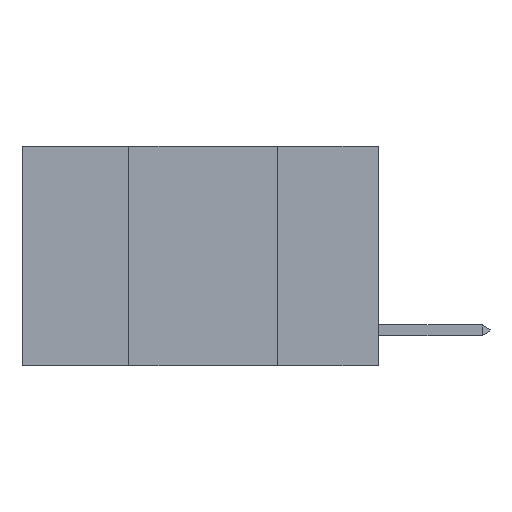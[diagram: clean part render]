
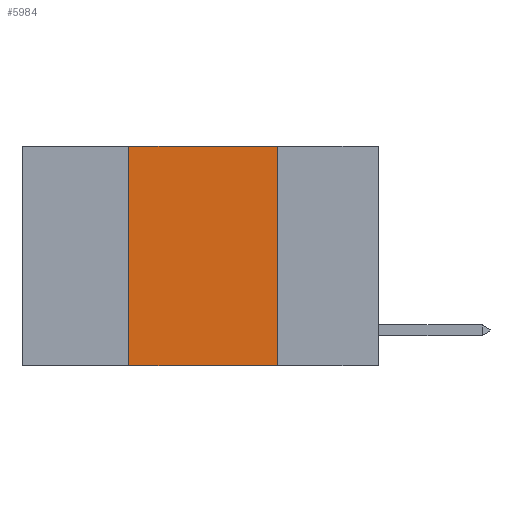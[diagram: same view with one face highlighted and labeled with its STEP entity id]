
A CAD part, left-side view. The second image highlights one B-rep face of the part: STEP entity #5984.
In plain terms, the highlighted planar face has unit normal (-1, 0, 0).
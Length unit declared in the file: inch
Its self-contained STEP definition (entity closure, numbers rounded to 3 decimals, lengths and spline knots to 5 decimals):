
#503 = DIRECTION ( 'NONE',  ( 0., 0., 1. ) ) ;
#614 = VECTOR ( 'NONE', #2839, 39.37008 ) ;
#666 = DIRECTION ( 'NONE',  ( 0., -1., 0. ) ) ;
#757 = CARTESIAN_POINT ( 'NONE',  ( 0., 0.6, 0. ) ) ;
#1487 = EDGE_CURVE ( 'NONE', #12241, #12350, #9036, .T. ) ;
#1735 = CARTESIAN_POINT ( 'NONE',  ( 0., 0.42, -0.37 ) ) ;
#2281 = LINE ( 'NONE', #3806, #614 ) ;
#2357 = VECTOR ( 'NONE', #666, 39.37008 ) ;
#2456 = DIRECTION ( 'NONE',  ( 0., -1., 0. ) ) ;
#2829 = CARTESIAN_POINT ( 'NONE',  ( 0., 0.42, 0. ) ) ;
#2839 = DIRECTION ( 'NONE',  ( 0., 0., -1. ) ) ;
#3806 = CARTESIAN_POINT ( 'NONE',  ( 0., 0.17, 0. ) ) ;
#3954 = EDGE_CURVE ( 'NONE', #12350, #12068, #5309, .T. ) ;
#4255 = FACE_OUTER_BOUND ( 'NONE', #10425, .T. ) ;
#4308 = VERTEX_POINT ( 'NONE', #11320 ) ;
#4888 = EDGE_CURVE ( 'NONE', #12241, #4308, #5291, .T. ) ;
#5291 = LINE ( 'NONE', #9980, #6110 ) ;
#5309 = LINE ( 'NONE', #10103, #2357 ) ;
#5984 = ADVANCED_FACE ( 'NONE', ( #4255 ), #13391, .F. ) ;
#6110 = VECTOR ( 'NONE', #2456, 39.37008 ) ;
#6283 = ORIENTED_EDGE ( 'NONE', *, *, #4888, .T. ) ;
#6851 = CARTESIAN_POINT ( 'NONE',  ( 0., 0.42, 0. ) ) ;
#6866 = VECTOR ( 'NONE', #503, 39.37008 ) ;
#7147 = ORIENTED_EDGE ( 'NONE', *, *, #1487, .F. ) ;
#9036 = LINE ( 'NONE', #6851, #6866 ) ;
#9254 = DIRECTION ( 'NONE',  ( 1., 0., 0. ) ) ;
#9519 = CARTESIAN_POINT ( 'NONE',  ( 0., 0.17, 0. ) ) ;
#9980 = CARTESIAN_POINT ( 'NONE',  ( 0., 0.6, -0.37 ) ) ;
#10103 = CARTESIAN_POINT ( 'NONE',  ( 0., 0.6, 0. ) ) ;
#10425 = EDGE_LOOP ( 'NONE', ( #12766, #12997, #7147, #6283 ) ) ;
#11320 = CARTESIAN_POINT ( 'NONE',  ( 0., 0.17, -0.37 ) ) ;
#11580 = EDGE_CURVE ( 'NONE', #12068, #4308, #2281, .T. ) ;
#12068 = VERTEX_POINT ( 'NONE', #9519 ) ;
#12241 = VERTEX_POINT ( 'NONE', #1735 ) ;
#12350 = VERTEX_POINT ( 'NONE', #2829 ) ;
#12766 = ORIENTED_EDGE ( 'NONE', *, *, #11580, .F. ) ;
#12997 = ORIENTED_EDGE ( 'NONE', *, *, #3954, .F. ) ;
#13005 = AXIS2_PLACEMENT_3D ( 'NONE', #757, #9254, #13251 ) ;
#13251 = DIRECTION ( 'NONE',  ( 0., 0., -1. ) ) ;
#13391 = PLANE ( 'NONE',  #13005 ) ;
